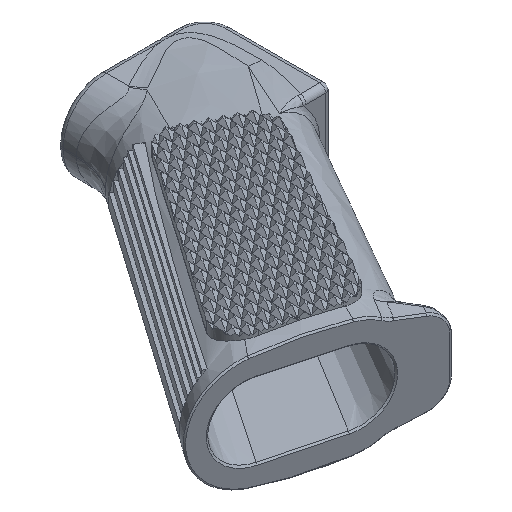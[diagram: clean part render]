
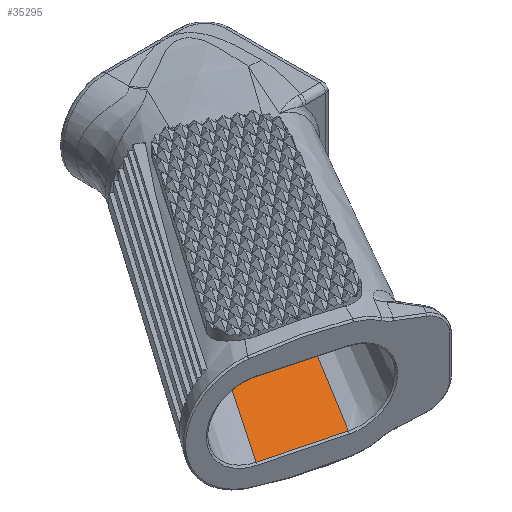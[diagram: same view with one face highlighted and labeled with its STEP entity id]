
A CAD part, isometric view. The second image highlights one B-rep face of the part: STEP entity #35295.
In plain terms, the highlighted planar face has unit normal (-0.01, -0.018, 1).
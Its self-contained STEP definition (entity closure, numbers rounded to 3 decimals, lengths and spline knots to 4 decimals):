
#46=PLANE($,#37728);
#2356=LINE($,#50405,#7106);
#2365=LINE($,#50571,#7115);
#2366=LINE($,#50601,#7116);
#7106=VECTOR($,#40298,1.9107);
#7115=VECTOR($,#40315,6.0505);
#7116=VECTOR($,#40316,5.9179);
#12084=B_SPLINE_CURVE_WITH_KNOTS($,3,(#50509,#50510,#50511,#50512,#50513,
#50514),.UNSPECIFIED.,.F.,.F.,(4,2,4),(0.,0.0058,0.0116),
 .UNSPECIFIED.);
#12087=B_SPLINE_CURVE_WITH_KNOTS($,3,(#50573,#50574,#50575,#50576),
 .UNSPECIFIED.,.F.,.F.,(4,4),(-6.3335,-6.2266),
 .UNSPECIFIED.);
#12088=B_SPLINE_CURVE_WITH_KNOTS($,3,(#50578,#50579,#50580,#50581,#50582,
#50583,#50584,#50585),.UNSPECIFIED.,.F.,.F.,(4,1,1,1,1,4),(-17.9216,
-16.6589,-14.1334,-11.608,-10.3453,
-9.0825),.UNSPECIFIED.);
#12089=B_SPLINE_CURVE_WITH_KNOTS($,3,(#50587,#50588,#50589,#50590),
 .UNSPECIFIED.,.F.,.F.,(4,4),(-19.013,-17.9216),
 .UNSPECIFIED.);
#12090=B_SPLINE_CURVE_WITH_KNOTS($,3,(#50592,#50593,#50594,#50595),
 .UNSPECIFIED.,.F.,.F.,(4,4),(3.6739,3.8042),
 .UNSPECIFIED.);
#12091=B_SPLINE_CURVE_WITH_KNOTS($,3,(#50597,#50598,#50599,#50600),
 .UNSPECIFIED.,.F.,.F.,(4,4),(2.4024,2.5218),
 .UNSPECIFIED.);
#12255=FACE_OUTER_BOUND($,#14687,.T.);
#14687=EDGE_LOOP($,(#25070,#25071,#25072,#25073,#25074,#25075,#25076,#25077,
#25078));
#17206=VERTEX_POINT($,#50398);
#17209=VERTEX_POINT($,#50403);
#17210=VERTEX_POINT($,#50467);
#17218=VERTEX_POINT($,#50570);
#17219=VERTEX_POINT($,#50572);
#17220=VERTEX_POINT($,#50577);
#17221=VERTEX_POINT($,#50586);
#17222=VERTEX_POINT($,#50591);
#17223=VERTEX_POINT($,#50596);
#19915=EDGE_CURVE($,#17209,#17206,#2356,.T.);
#19922=EDGE_CURVE($,#17210,#17209,#12084,.T.);
#19932=EDGE_CURVE($,#17218,#17210,#2365,.T.);
#19933=EDGE_CURVE($,#17219,#17218,#12087,.T.);
#19934=EDGE_CURVE($,#17220,#17219,#12088,.T.);
#19935=EDGE_CURVE($,#17221,#17220,#12089,.T.);
#19936=EDGE_CURVE($,#17222,#17221,#12090,.T.);
#19937=EDGE_CURVE($,#17223,#17222,#12091,.T.);
#19938=EDGE_CURVE($,#17206,#17223,#2366,.T.);
#25070=ORIENTED_EDGE($,*,*,#19915,.F.);
#25071=ORIENTED_EDGE($,*,*,#19922,.F.);
#25072=ORIENTED_EDGE($,*,*,#19932,.F.);
#25073=ORIENTED_EDGE($,*,*,#19933,.F.);
#25074=ORIENTED_EDGE($,*,*,#19934,.F.);
#25075=ORIENTED_EDGE($,*,*,#19935,.F.);
#25076=ORIENTED_EDGE($,*,*,#19936,.F.);
#25077=ORIENTED_EDGE($,*,*,#19937,.F.);
#25078=ORIENTED_EDGE($,*,*,#19938,.F.);
#35295=ADVANCED_FACE($,(#12255),#46,.T.);
#37728=AXIS2_PLACEMENT_3D($,#50569,#40313,#40314);
#40298=DIRECTION($,(-0.966,0.259,-0.005));
#40313=DIRECTION('center_axis',(-0.01,-0.018,
1.));
#40314=DIRECTION('ref_axis',(1.,0.,0.01));
#40315=DIRECTION($,(-0.517,-0.856,-0.02));
#40316=DIRECTION($,(0.557,0.83,0.02));
#50398=CARTESIAN_POINT('',(-20.6217,-11.3394,-0.8454));
#50403=CARTESIAN_POINT('',(-18.7761,-11.8339,-0.8353));
#50405=CARTESIAN_POINT($,(-18.7792,-11.8331,-0.8354));
#50467=CARTESIAN_POINT('',(-18.7649,-11.8369,-0.8353));
#50509=CARTESIAN_POINT('Ctrl Pts',(-18.7649,-11.8369,
-0.8353));
#50510=CARTESIAN_POINT('Ctrl Pts',(-18.7667,-11.8364,
-0.8353));
#50511=CARTESIAN_POINT('Ctrl Pts',(-18.7686,-11.8359,-0.8353));
#50512=CARTESIAN_POINT('Ctrl Pts',(-18.7723,-11.8349,
-0.8353));
#50513=CARTESIAN_POINT('Ctrl Pts',(-18.7742,-11.8344,
-0.8353));
#50514=CARTESIAN_POINT('Ctrl Pts',(-18.7761,-11.8339,
-0.8353));
#50569=CARTESIAN_POINT('Origin',(-17.9239,-8.8083,-0.7734));
#50570=CARTESIAN_POINT('',(-15.6344,-6.6607,-0.7124));
#50571=CARTESIAN_POINT($,(-15.0029,-5.6164,-0.6876));
#50572=CARTESIAN_POINT('',(-15.7072,-6.5669,-0.7115));
#50573=CARTESIAN_POINT('Ctrl Pts',(-15.7072,-6.5669,
-0.7115));
#50574=CARTESIAN_POINT('Ctrl Pts',(-15.6833,-6.5984,
-0.7118));
#50575=CARTESIAN_POINT('Ctrl Pts',(-15.6591,-6.6296,
-0.7121));
#50576=CARTESIAN_POINT('Ctrl Pts',(-15.6344,-6.6607,
-0.7124));
#50577=CARTESIAN_POINT('',(-16.6986,-6.3332,-0.7174));
#50578=CARTESIAN_POINT('Ctrl Pts',(-16.6986,-6.3332,-0.7174));
#50579=CARTESIAN_POINT('Ctrl Pts',(-16.5843,-6.3192,
-0.716));
#50580=CARTESIAN_POINT('Ctrl Pts',(-16.3051,-6.2962,-0.7128));
#50581=CARTESIAN_POINT('Ctrl Pts',(-16.0381,-6.3226,
-0.7105));
#50582=CARTESIAN_POINT('Ctrl Pts',(-15.8972,-6.3834,
-0.7102));
#50583=CARTESIAN_POINT('Ctrl Pts',(-15.7936,-6.4642,
-0.7105));
#50584=CARTESIAN_POINT('Ctrl Pts',(-15.7372,-6.5272,
-0.7111));
#50585=CARTESIAN_POINT('Ctrl Pts',(-15.7072,-6.5669,
-0.7115));
#50586=CARTESIAN_POINT('',(-17.0515,-6.3864,-0.7219));
#50587=CARTESIAN_POINT('Ctrl Pts',(-17.0515,-6.3864,
-0.7219));
#50588=CARTESIAN_POINT('Ctrl Pts',(-16.9119,-6.3622,
-0.7201));
#50589=CARTESIAN_POINT('Ctrl Pts',(-16.7974,-6.3453,-0.7186));
#50590=CARTESIAN_POINT('Ctrl Pts',(-16.6986,-6.3332,-0.7174));
#50591=CARTESIAN_POINT('',(-17.1922,-6.4089,-0.7238));
#50592=CARTESIAN_POINT('Ctrl Pts',(-17.1922,-6.4089,
-0.7238));
#50593=CARTESIAN_POINT('Ctrl Pts',(-17.1453,-6.4021,
-0.7232));
#50594=CARTESIAN_POINT('Ctrl Pts',(-17.0985,-6.3946,
-0.7226));
#50595=CARTESIAN_POINT('Ctrl Pts',(-17.0515,-6.3864,
-0.7219));
#50596=CARTESIAN_POINT('',(-17.3268,-6.425,-0.7254));
#50597=CARTESIAN_POINT('Ctrl Pts',(-17.3268,-6.425,-0.7254));
#50598=CARTESIAN_POINT('Ctrl Pts',(-17.2807,-6.4209,
-0.7249));
#50599=CARTESIAN_POINT('Ctrl Pts',(-17.2359,-6.4153,
-0.7243));
#50600=CARTESIAN_POINT('Ctrl Pts',(-17.1922,-6.4089,
-0.7238));
#50601=CARTESIAN_POINT($,(-20.8515,-11.6822,-0.8538));
